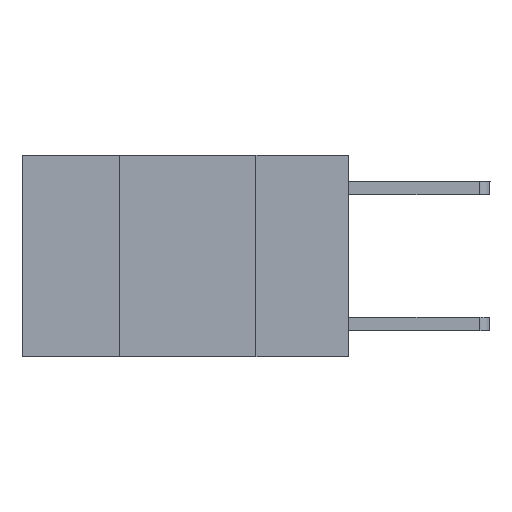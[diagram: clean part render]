
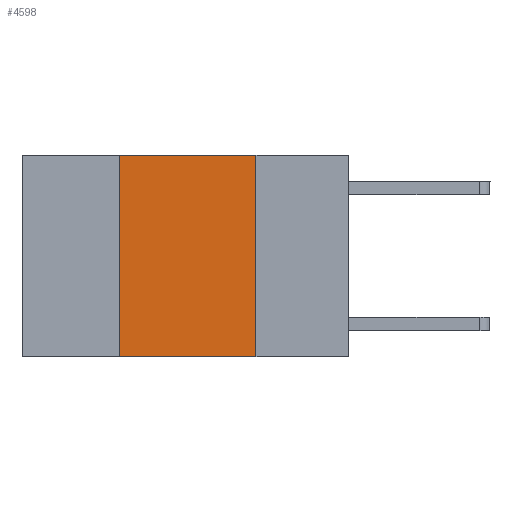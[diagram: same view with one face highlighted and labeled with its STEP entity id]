
A CAD part, left-side view. The second image highlights one B-rep face of the part: STEP entity #4598.
In plain terms, the highlighted planar face has unit normal (-1, 0, 0).
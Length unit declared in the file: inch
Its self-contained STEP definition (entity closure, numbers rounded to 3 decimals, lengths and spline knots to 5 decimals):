
#150 = CARTESIAN_POINT ( 'NONE',  ( 0., 0.6, -0.37 ) ) ;
#532 = VECTOR ( 'NONE', #9036, 39.37008 ) ;
#1390 = ORIENTED_EDGE ( 'NONE', *, *, #3662, .F. ) ;
#1475 = ORIENTED_EDGE ( 'NONE', *, *, #8286, .F. ) ;
#1705 = CARTESIAN_POINT ( 'NONE',  ( 0., 0.6, 0. ) ) ;
#2122 = ORIENTED_EDGE ( 'NONE', *, *, #2342, .T. ) ;
#2334 = ORIENTED_EDGE ( 'NONE', *, *, #6473, .F. ) ;
#2342 = EDGE_CURVE ( 'NONE', #3810, #3977, #2475, .T. ) ;
#2475 = LINE ( 'NONE', #150, #532 ) ;
#2545 = CARTESIAN_POINT ( 'NONE',  ( 0., 0.17, 0. ) ) ;
#2613 = VERTEX_POINT ( 'NONE', #4787 ) ;
#2765 = EDGE_LOOP ( 'NONE', ( #1390, #1475, #2334, #2122 ) ) ;
#2822 = VERTEX_POINT ( 'NONE', #2545 ) ;
#2918 = VECTOR ( 'NONE', #7392, 39.37008 ) ;
#3028 = AXIS2_PLACEMENT_3D ( 'NONE', #3580, #3305, #3283 ) ;
#3283 = DIRECTION ( 'NONE',  ( 0., 0., -1. ) ) ;
#3305 = DIRECTION ( 'NONE',  ( 1., 0., 0. ) ) ;
#3321 = PLANE ( 'NONE',  #3028 ) ;
#3580 = CARTESIAN_POINT ( 'NONE',  ( 0., 0.6, 0. ) ) ;
#3662 = EDGE_CURVE ( 'NONE', #2822, #3977, #8753, .T. ) ;
#3810 = VERTEX_POINT ( 'NONE', #6647 ) ;
#3977 = VERTEX_POINT ( 'NONE', #5954 ) ;
#4491 = DIRECTION ( 'NONE',  ( 0., 0., 1. ) ) ;
#4598 = ADVANCED_FACE ( 'NONE', ( #5607 ), #3321, .F. ) ;
#4787 = CARTESIAN_POINT ( 'NONE',  ( 0., 0.42, 0. ) ) ;
#4960 = VECTOR ( 'NONE', #5345, 39.37008 ) ;
#5345 = DIRECTION ( 'NONE',  ( 0., -1., 0. ) ) ;
#5607 = FACE_OUTER_BOUND ( 'NONE', #2765, .T. ) ;
#5954 = CARTESIAN_POINT ( 'NONE',  ( 0., 0.17, -0.37 ) ) ;
#6254 = VECTOR ( 'NONE', #4491, 39.37008 ) ;
#6473 = EDGE_CURVE ( 'NONE', #3810, #2613, #8460, .T. ) ;
#6647 = CARTESIAN_POINT ( 'NONE',  ( 0., 0.42, -0.37 ) ) ;
#6696 = CARTESIAN_POINT ( 'NONE',  ( 0., 0.42, 0. ) ) ;
#7332 = CARTESIAN_POINT ( 'NONE',  ( 0., 0.17, 0. ) ) ;
#7392 = DIRECTION ( 'NONE',  ( 0., 0., -1. ) ) ;
#8286 = EDGE_CURVE ( 'NONE', #2613, #2822, #8637, .T. ) ;
#8460 = LINE ( 'NONE', #6696, #6254 ) ;
#8637 = LINE ( 'NONE', #1705, #4960 ) ;
#8753 = LINE ( 'NONE', #7332, #2918 ) ;
#9036 = DIRECTION ( 'NONE',  ( 0., -1., 0. ) ) ;
